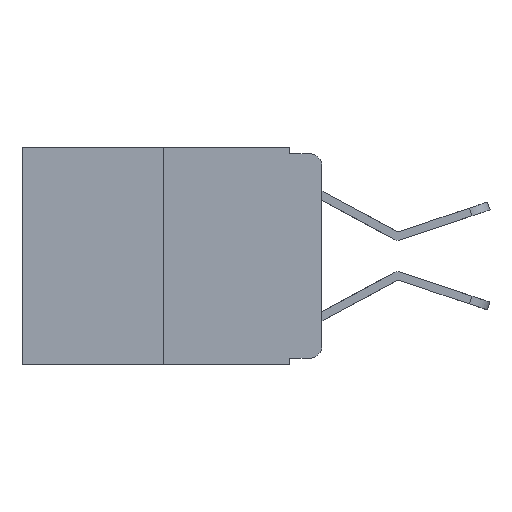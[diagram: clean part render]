
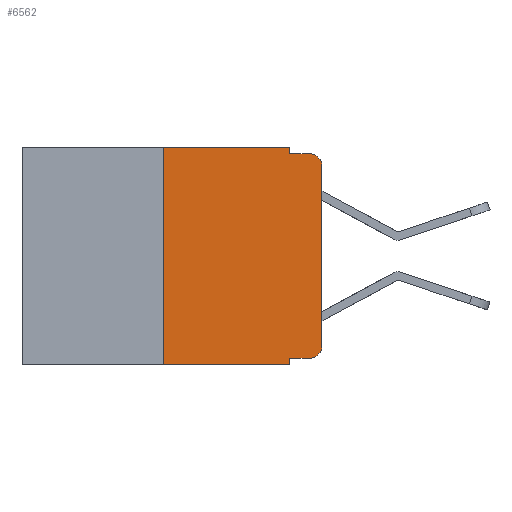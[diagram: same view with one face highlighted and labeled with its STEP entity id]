
A CAD part, left-side view. The second image highlights one B-rep face of the part: STEP entity #6562.
In plain terms, the highlighted planar face has unit normal (-1, 0, 0).
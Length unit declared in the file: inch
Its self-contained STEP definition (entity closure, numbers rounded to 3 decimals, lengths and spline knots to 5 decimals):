
#755 = DIRECTION ( 'NONE',  ( 0., 0., -1. ) ) ;
#1118 = LINE ( 'NONE', #12762, #12602 ) ;
#1278 = ORIENTED_EDGE ( 'NONE', *, *, #8615, .F. ) ;
#1365 = DIRECTION ( 'NONE',  ( 0., -1., 0. ) ) ;
#1525 = DIRECTION ( 'NONE',  ( 0., 0., -1. ) ) ;
#1683 = VECTOR ( 'NONE', #6204, 39.37008 ) ;
#1743 = CARTESIAN_POINT ( 'NONE',  ( 0., 0.02, -0.313 ) ) ;
#1927 = EDGE_CURVE ( 'NONE', #3985, #6970, #9349, .T. ) ;
#2080 = LINE ( 'NONE', #7318, #1683 ) ;
#2206 = CARTESIAN_POINT ( 'NONE',  ( 0., 0.02, -0.01 ) ) ;
#2276 = DIRECTION ( 'NONE',  ( 0., 0., 1. ) ) ;
#2587 = LINE ( 'NONE', #11470, #14298 ) ;
#2610 = ORIENTED_EDGE ( 'NONE', *, *, #10659, .F. ) ;
#2817 = VERTEX_POINT ( 'NONE', #11440 ) ;
#2927 = DIRECTION ( 'NONE',  ( 0., 0., -1. ) ) ;
#3290 = EDGE_CURVE ( 'NONE', #3985, #2817, #6253, .T. ) ;
#3658 = CARTESIAN_POINT ( 'NONE',  ( 0., 0.051, 0. ) ) ;
#3872 = PLANE ( 'NONE',  #6595 ) ;
#3985 = VERTEX_POINT ( 'NONE', #10330 ) ;
#4226 = LINE ( 'NONE', #7590, #12879 ) ;
#4611 = VERTEX_POINT ( 'NONE', #2206 ) ;
#5010 = CARTESIAN_POINT ( 'NONE',  ( 0., 0.473, 0. ) ) ;
#5300 = ORIENTED_EDGE ( 'NONE', *, *, #6119, .T. ) ;
#5504 = EDGE_LOOP ( 'NONE', ( #6880, #5300, #2610, #12743, #1278, #11571, #8860, #11921, #6892, #13269 ) ) ;
#6119 = EDGE_CURVE ( 'NONE', #12913, #4611, #12430, .T. ) ;
#6173 = CARTESIAN_POINT ( 'NONE',  ( 0., 0., -0.03 ) ) ;
#6204 = DIRECTION ( 'NONE',  ( 0., -1., 0. ) ) ;
#6253 = LINE ( 'NONE', #6805, #8938 ) ;
#6256 = EDGE_CURVE ( 'NONE', #11048, #12913, #9952, .T. ) ;
#6289 = VECTOR ( 'NONE', #11187, 39.37008 ) ;
#6409 = VERTEX_POINT ( 'NONE', #3658 ) ;
#6562 = ADVANCED_FACE ( 'NONE', ( #12748 ), #3872, .F. ) ;
#6595 = AXIS2_PLACEMENT_3D ( 'NONE', #5010, #8399, #1525 ) ;
#6805 = CARTESIAN_POINT ( 'NONE',  ( 0., 0.25, 0. ) ) ;
#6880 = ORIENTED_EDGE ( 'NONE', *, *, #6256, .T. ) ;
#6892 = ORIENTED_EDGE ( 'NONE', *, *, #11280, .T. ) ;
#6900 = VECTOR ( 'NONE', #2276, 39.37008 ) ;
#6970 = VERTEX_POINT ( 'NONE', #12703 ) ;
#6973 = CARTESIAN_POINT ( 'NONE',  ( 0., 0.02, -0.333 ) ) ;
#7318 = CARTESIAN_POINT ( 'NONE',  ( 0., 0.051, -0.333 ) ) ;
#7474 = EDGE_CURVE ( 'NONE', #11964, #6970, #2587, .T. ) ;
#7590 = CARTESIAN_POINT ( 'NONE',  ( 0., 0.051, 0. ) ) ;
#7683 = DIRECTION ( 'NONE',  ( -1., 0., 0. ) ) ;
#7933 = CARTESIAN_POINT ( 'NONE',  ( 0., 0., 0. ) ) ;
#8282 = DIRECTION ( 'NONE',  ( 0., -1., 0. ) ) ;
#8399 = DIRECTION ( 'NONE',  ( 1., 0., 0. ) ) ;
#8615 = EDGE_CURVE ( 'NONE', #2817, #6409, #13015, .T. ) ;
#8860 = ORIENTED_EDGE ( 'NONE', *, *, #1927, .T. ) ;
#8938 = VECTOR ( 'NONE', #14699, 39.37008 ) ;
#9241 = VERTEX_POINT ( 'NONE', #13972 ) ;
#9349 = LINE ( 'NONE', #10028, #6289 ) ;
#9549 = CARTESIAN_POINT ( 'NONE',  ( 0., 0.051, -0.333 ) ) ;
#9782 = DIRECTION ( 'NONE',  ( -1., 0., 0. ) ) ;
#9952 = LINE ( 'NONE', #7933, #6900 ) ;
#10028 = CARTESIAN_POINT ( 'NONE',  ( 0., 0.473, -0.343 ) ) ;
#10330 = CARTESIAN_POINT ( 'NONE',  ( 0., 0.25, -0.343 ) ) ;
#10643 = CARTESIAN_POINT ( 'NONE',  ( 0., 0.473, 0. ) ) ;
#10659 = EDGE_CURVE ( 'NONE', #9241, #4611, #1118, .T. ) ;
#11048 = VERTEX_POINT ( 'NONE', #12560 ) ;
#11187 = DIRECTION ( 'NONE',  ( 0., -1., 0. ) ) ;
#11280 = EDGE_CURVE ( 'NONE', #11964, #12723, #2080, .T. ) ;
#11440 = CARTESIAN_POINT ( 'NONE',  ( 0., 0.25, 0. ) ) ;
#11470 = CARTESIAN_POINT ( 'NONE',  ( 0., 0.051, 0. ) ) ;
#11571 = ORIENTED_EDGE ( 'NONE', *, *, #3290, .F. ) ;
#11921 = ORIENTED_EDGE ( 'NONE', *, *, #7474, .F. ) ;
#11964 = VERTEX_POINT ( 'NONE', #9549 ) ;
#12202 = CIRCLE ( 'NONE', #13592, 0.02 ) ;
#12228 = DIRECTION ( 'NONE',  ( 0., 0., -1. ) ) ;
#12430 = CIRCLE ( 'NONE', #13224, 0.02 ) ;
#12560 = CARTESIAN_POINT ( 'NONE',  ( 0., 0., -0.313 ) ) ;
#12602 = VECTOR ( 'NONE', #1365, 39.37008 ) ;
#12670 = VECTOR ( 'NONE', #8282, 39.37008 ) ;
#12703 = CARTESIAN_POINT ( 'NONE',  ( 0., 0.051, -0.343 ) ) ;
#12723 = VERTEX_POINT ( 'NONE', #6973 ) ;
#12743 = ORIENTED_EDGE ( 'NONE', *, *, #14279, .F. ) ;
#12748 = FACE_OUTER_BOUND ( 'NONE', #5504, .T. ) ;
#12762 = CARTESIAN_POINT ( 'NONE',  ( 0., 0.051, -0.01 ) ) ;
#12879 = VECTOR ( 'NONE', #12228, 39.37008 ) ;
#12913 = VERTEX_POINT ( 'NONE', #6173 ) ;
#13015 = LINE ( 'NONE', #10643, #12670 ) ;
#13224 = AXIS2_PLACEMENT_3D ( 'NONE', #14496, #7683, #755 ) ;
#13269 = ORIENTED_EDGE ( 'NONE', *, *, #14911, .T. ) ;
#13592 = AXIS2_PLACEMENT_3D ( 'NONE', #1743, #9782, #2927 ) ;
#13972 = CARTESIAN_POINT ( 'NONE',  ( 0., 0.051, -0.01 ) ) ;
#14279 = EDGE_CURVE ( 'NONE', #6409, #9241, #4226, .T. ) ;
#14298 = VECTOR ( 'NONE', #14803, 39.37008 ) ;
#14496 = CARTESIAN_POINT ( 'NONE',  ( 0., 0.02, -0.03 ) ) ;
#14699 = DIRECTION ( 'NONE',  ( 0., 0., 1. ) ) ;
#14803 = DIRECTION ( 'NONE',  ( 0., 0., -1. ) ) ;
#14911 = EDGE_CURVE ( 'NONE', #12723, #11048, #12202, .T. ) ;
